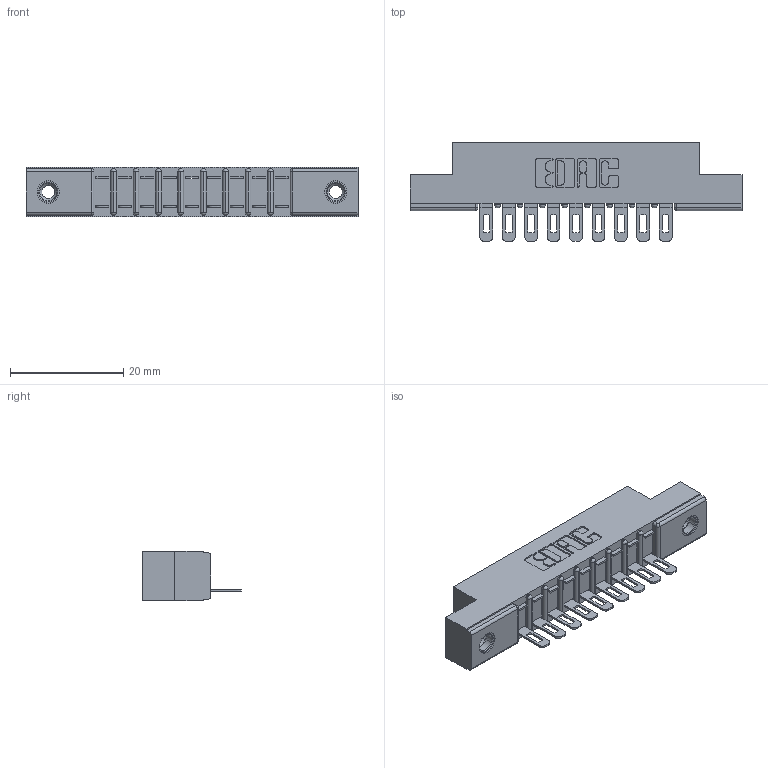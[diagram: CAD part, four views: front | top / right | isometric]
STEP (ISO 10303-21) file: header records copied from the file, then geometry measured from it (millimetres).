
FILE_DESCRIPTION (( 'STEP AP203' ), '1' );
FILE_NAME ('357-009-501-108.STEP', '2018-08-07T01:58:30', ( '' ), ( '' ), 'SwSTEP 2.0', 'SolidWorks 2016', '' );
FILE_SCHEMA (( 'CONFIG_CONTROL_DESIGN' ));
Length unit declared in the file: inch
Products named in the file (4): 307 Part_.156 Dia Mounting Holes; 307-290-002_501; 345-250-001_345-250-003-102; 357-009-501-108
Assembly tree (12 placements, depth 2):
  357-009-501-108
    307 Part_.156 Dia Mounting Holes
    307-290-002_501  x9
    345-250-001_345-250-003-102  x2
Bounding box: 58.67 x 17.42 x 8.71 mm (x, y, z)
Volume: 3868.1 mm3; surface area: 6391.8 mm2
Topology: 12 solids, 12 shells, 872 faces, 2601 edges, 1698 vertices
Faces by surface type: plane 498, cylinder 338, sphere 20, cone 12, torus 4
Entity records: 13763 total; most frequent: CARTESIAN_POINT 2295, ORIENTED_EDGE 2278, DIRECTION 2259, EDGE_CURVE 1139, LINE 851, VECTOR 851, VERTEX_POINT 740, AXIS2_PLACEMENT_3D 704
